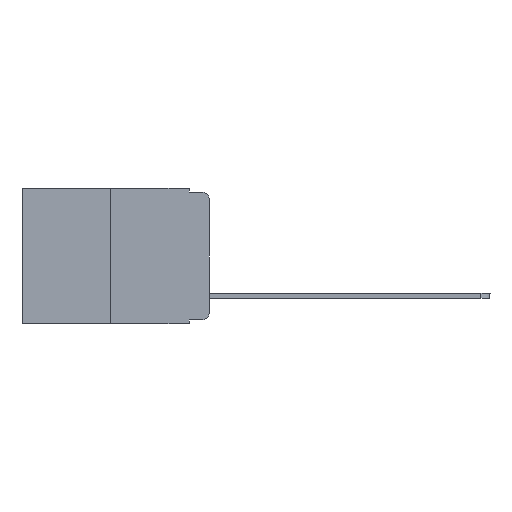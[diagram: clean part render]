
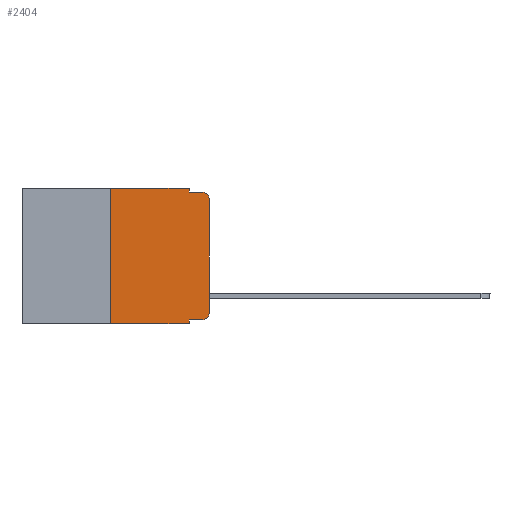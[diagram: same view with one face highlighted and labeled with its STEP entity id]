
A CAD part, left-side view. The second image highlights one B-rep face of the part: STEP entity #2404.
In plain terms, the highlighted planar face has unit normal (-1, 0, 0).
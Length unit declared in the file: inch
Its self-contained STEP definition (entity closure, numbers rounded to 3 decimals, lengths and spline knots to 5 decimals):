
#218 = LINE ( 'NONE', #775, #11002 ) ;
#280 = CARTESIAN_POINT ( 'NONE',  ( 0., 0.473, 0. ) ) ;
#308 = DIRECTION ( 'NONE',  ( 0., 0., -1. ) ) ;
#421 = EDGE_CURVE ( 'NONE', #429, #1758, #5145, .T. ) ;
#429 = VERTEX_POINT ( 'NONE', #6295 ) ;
#703 = ORIENTED_EDGE ( 'NONE', *, *, #10820, .T. ) ;
#775 = CARTESIAN_POINT ( 'NONE',  ( 0., 0.25, 0. ) ) ;
#970 = CIRCLE ( 'NONE', #9754, 0.02 ) ;
#1045 = CARTESIAN_POINT ( 'NONE',  ( 0., 0.051, 0. ) ) ;
#1245 = EDGE_LOOP ( 'NONE', ( #12214, #12792, #3099, #5261, #10171, #12622, #8104, #3011, #9389, #703 ) ) ;
#1352 = FACE_OUTER_BOUND ( 'NONE', #1245, .T. ) ;
#1534 = VERTEX_POINT ( 'NONE', #7800 ) ;
#1663 = DIRECTION ( 'NONE',  ( -1., 0., 0. ) ) ;
#1758 = VERTEX_POINT ( 'NONE', #8374 ) ;
#2281 = LINE ( 'NONE', #4154, #6177 ) ;
#2404 = ADVANCED_FACE ( 'NONE', ( #1352 ), #12627, .F. ) ;
#2428 = VECTOR ( 'NONE', #6096, 39.37008 ) ;
#2591 = CARTESIAN_POINT ( 'NONE',  ( 0., 0.473, 0. ) ) ;
#2919 = VECTOR ( 'NONE', #12758, 39.37008 ) ;
#3011 = ORIENTED_EDGE ( 'NONE', *, *, #4774, .F. ) ;
#3099 = ORIENTED_EDGE ( 'NONE', *, *, #3449, .F. ) ;
#3176 = VECTOR ( 'NONE', #4865, 39.37008 ) ;
#3256 = DIRECTION ( 'NONE',  ( 0., -1., 0. ) ) ;
#3449 = EDGE_CURVE ( 'NONE', #10944, #4015, #2281, .T. ) ;
#3458 = VERTEX_POINT ( 'NONE', #12460 ) ;
#4015 = VERTEX_POINT ( 'NONE', #11223 ) ;
#4154 = CARTESIAN_POINT ( 'NONE',  ( 0., 0.051, -0.01 ) ) ;
#4234 = VERTEX_POINT ( 'NONE', #12530 ) ;
#4246 = CARTESIAN_POINT ( 'NONE',  ( 0., 0.051, 0. ) ) ;
#4261 = DIRECTION ( 'NONE',  ( -1., 0., 0. ) ) ;
#4280 = DIRECTION ( 'NONE',  ( 0., -1., 0. ) ) ;
#4538 = EDGE_CURVE ( 'NONE', #1758, #10944, #5077, .T. ) ;
#4576 = DIRECTION ( 'NONE',  ( 0., 0., -1. ) ) ;
#4706 = EDGE_CURVE ( 'NONE', #9726, #1534, #8215, .T. ) ;
#4752 = LINE ( 'NONE', #4246, #6649 ) ;
#4774 = EDGE_CURVE ( 'NONE', #3458, #1534, #4752, .T. ) ;
#4809 = CIRCLE ( 'NONE', #10627, 0.02 ) ;
#4865 = DIRECTION ( 'NONE',  ( 0., -1., 0. ) ) ;
#5077 = LINE ( 'NONE', #1045, #2428 ) ;
#5145 = LINE ( 'NONE', #280, #8787 ) ;
#5247 = DIRECTION ( 'NONE',  ( 0., 0., -1. ) ) ;
#5261 = ORIENTED_EDGE ( 'NONE', *, *, #4538, .F. ) ;
#5314 = DIRECTION ( 'NONE',  ( 0., -1., 0. ) ) ;
#5371 = VECTOR ( 'NONE', #3256, 39.37008 ) ;
#5374 = AXIS2_PLACEMENT_3D ( 'NONE', #2591, #5488, #4576 ) ;
#5483 = EDGE_CURVE ( 'NONE', #9726, #429, #218, .T. ) ;
#5488 = DIRECTION ( 'NONE',  ( 1., 0., 0. ) ) ;
#5570 = DIRECTION ( 'NONE',  ( 0., 0., -1. ) ) ;
#5617 = CARTESIAN_POINT ( 'NONE',  ( 0., 0.051, -0.01 ) ) ;
#5897 = CARTESIAN_POINT ( 'NONE',  ( 0., 0.25, -0.343 ) ) ;
#6096 = DIRECTION ( 'NONE',  ( 0., 0., -1. ) ) ;
#6177 = VECTOR ( 'NONE', #4280, 39.37008 ) ;
#6270 = CARTESIAN_POINT ( 'NONE',  ( 0., 0., -0.313 ) ) ;
#6295 = CARTESIAN_POINT ( 'NONE',  ( 0., 0.25, 0. ) ) ;
#6373 = CARTESIAN_POINT ( 'NONE',  ( 0., 0., -0.03 ) ) ;
#6649 = VECTOR ( 'NONE', #5247, 39.37008 ) ;
#7103 = VERTEX_POINT ( 'NONE', #6270 ) ;
#7288 = LINE ( 'NONE', #12440, #2919 ) ;
#7329 = CARTESIAN_POINT ( 'NONE',  ( 0., 0.473, -0.343 ) ) ;
#7409 = EDGE_CURVE ( 'NONE', #3458, #4234, #11004, .T. ) ;
#7605 = CARTESIAN_POINT ( 'NONE',  ( 0., 0.02, -0.313 ) ) ;
#7800 = CARTESIAN_POINT ( 'NONE',  ( 0., 0.051, -0.343 ) ) ;
#8104 = ORIENTED_EDGE ( 'NONE', *, *, #4706, .T. ) ;
#8215 = LINE ( 'NONE', #7329, #5371 ) ;
#8374 = CARTESIAN_POINT ( 'NONE',  ( 0., 0.051, 0. ) ) ;
#8653 = EDGE_CURVE ( 'NONE', #10470, #4015, #970, .T. ) ;
#8787 = VECTOR ( 'NONE', #5314, 39.37008 ) ;
#9389 = ORIENTED_EDGE ( 'NONE', *, *, #7409, .T. ) ;
#9467 = DIRECTION ( 'NONE',  ( 0., 0., 1. ) ) ;
#9726 = VERTEX_POINT ( 'NONE', #5897 ) ;
#9754 = AXIS2_PLACEMENT_3D ( 'NONE', #10252, #4261, #308 ) ;
#10171 = ORIENTED_EDGE ( 'NONE', *, *, #421, .F. ) ;
#10252 = CARTESIAN_POINT ( 'NONE',  ( 0., 0.02, -0.03 ) ) ;
#10470 = VERTEX_POINT ( 'NONE', #6373 ) ;
#10627 = AXIS2_PLACEMENT_3D ( 'NONE', #7605, #1663, #5570 ) ;
#10820 = EDGE_CURVE ( 'NONE', #4234, #7103, #4809, .T. ) ;
#10944 = VERTEX_POINT ( 'NONE', #5617 ) ;
#10994 = CARTESIAN_POINT ( 'NONE',  ( 0., 0.051, -0.333 ) ) ;
#11002 = VECTOR ( 'NONE', #9467, 39.37008 ) ;
#11004 = LINE ( 'NONE', #10994, #3176 ) ;
#11223 = CARTESIAN_POINT ( 'NONE',  ( 0., 0.02, -0.01 ) ) ;
#12214 = ORIENTED_EDGE ( 'NONE', *, *, #12811, .T. ) ;
#12440 = CARTESIAN_POINT ( 'NONE',  ( 0., 0., 0. ) ) ;
#12460 = CARTESIAN_POINT ( 'NONE',  ( 0., 0.051, -0.333 ) ) ;
#12530 = CARTESIAN_POINT ( 'NONE',  ( 0., 0.02, -0.333 ) ) ;
#12622 = ORIENTED_EDGE ( 'NONE', *, *, #5483, .F. ) ;
#12627 = PLANE ( 'NONE',  #5374 ) ;
#12758 = DIRECTION ( 'NONE',  ( 0., 0., 1. ) ) ;
#12792 = ORIENTED_EDGE ( 'NONE', *, *, #8653, .T. ) ;
#12811 = EDGE_CURVE ( 'NONE', #7103, #10470, #7288, .T. ) ;
